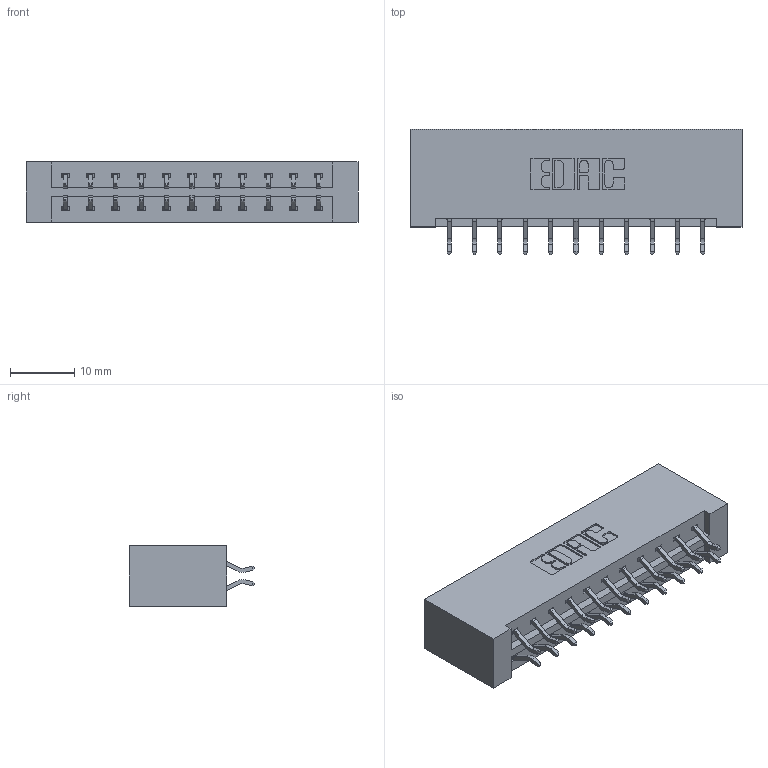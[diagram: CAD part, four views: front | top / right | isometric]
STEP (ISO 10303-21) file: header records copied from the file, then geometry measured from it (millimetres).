
FILE_DESCRIPTION (( 'STEP AP203' ), '1' );
FILE_NAME ('333-022-556-201.STEP', '2018-08-02T02:41:07', ( '' ), ( '' ), 'SwSTEP 2.0', 'SolidWorks 2016', '' );
FILE_SCHEMA (( 'CONFIG_CONTROL_DESIGN' ));
Length unit declared in the file: inch
Products named in the file (3): 333 Part_Lugless; 345-292-001_556 Tail; 333-022-556-201
Assembly tree (23 placements, depth 2):
  333-022-556-201
    333 Part_Lugless
    345-292-001_556 Tail  x22
Bounding box: 51.84 x 19.57 x 9.4 mm (x, y, z)
Volume: 5634.2 mm3; surface area: 6330.5 mm2
Topology: 23 solids, 23 shells, 1382 faces, 4093 edges, 2698 vertices
Faces by surface type: plane 946, cylinder 436
Entity records: 11029 total; most frequent: CARTESIAN_POINT 1878, ORIENTED_EDGE 1802, DIRECTION 1641, EDGE_CURVE 901, LINE 773, VECTOR 773, VERTEX_POINT 598, AXIS2_PLACEMENT_3D 434
